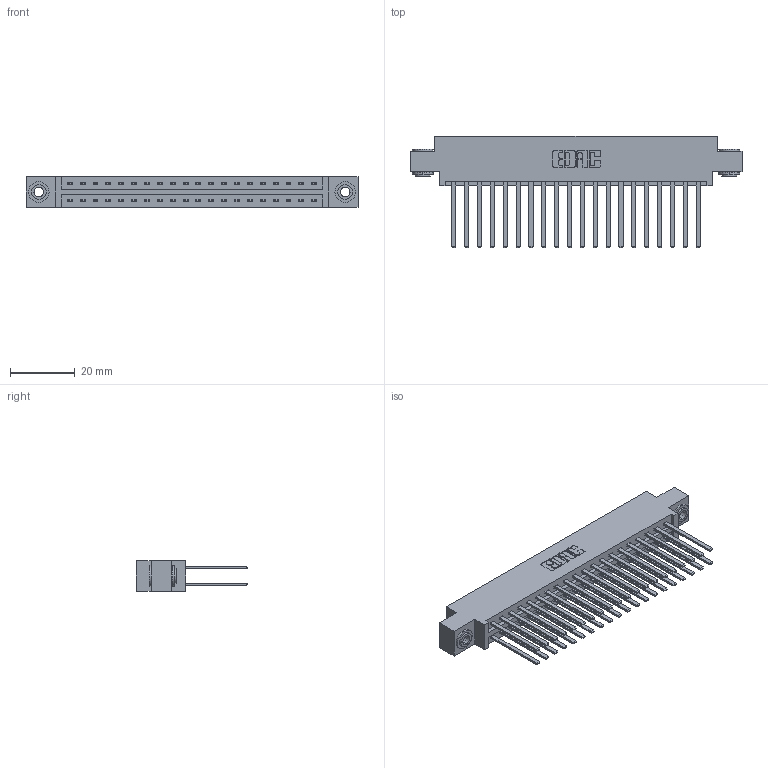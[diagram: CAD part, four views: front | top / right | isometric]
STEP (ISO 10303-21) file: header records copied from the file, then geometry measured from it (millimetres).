
FILE_DESCRIPTION (( 'STEP AP203' ), '1' );
FILE_NAME ('387-040-544-803.STEP', '2018-09-19T16:46:25', ( '' ), ( '' ), 'SwSTEP 2.0', 'SolidWorks 2016', '' );
FILE_SCHEMA (( 'CONFIG_CONTROL_DESIGN' ));
Length unit declared in the file: inch
Products named in the file (4): 337 Part_0.170 Offset - 0.156 Dia-TH; 345-292-001_345-293-144; 345-250-002_345-250-002-102; 387-040-544-803
Assembly tree (43 placements, depth 2):
  387-040-544-803
    337 Part_0.170 Offset - 0.156 Dia-TH
    345-292-001_345-293-144  x40
    345-250-002_345-250-002-102  x2
Bounding box: 102.26 x 34.3 x 9.4 mm (x, y, z)
Volume: 10946.8 mm3; surface area: 14325.6 mm2
Topology: 43 solids, 43 shells, 2076 faces, 6119 edges, 4022 vertices
Faces by surface type: plane 1444, cylinder 624, cone 8
Entity records: 18950 total; most frequent: CARTESIAN_POINT 3185, ORIENTED_EDGE 3114, DIRECTION 2779, EDGE_CURVE 1557, VECTOR 1409, LINE 1409, VERTEX_POINT 1034, AXIS2_PLACEMENT_3D 685
